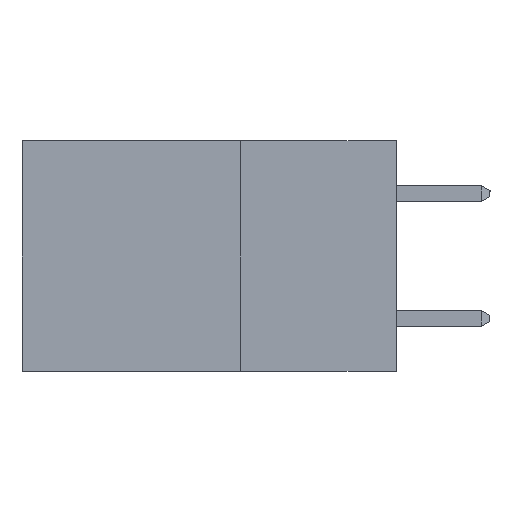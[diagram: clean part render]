
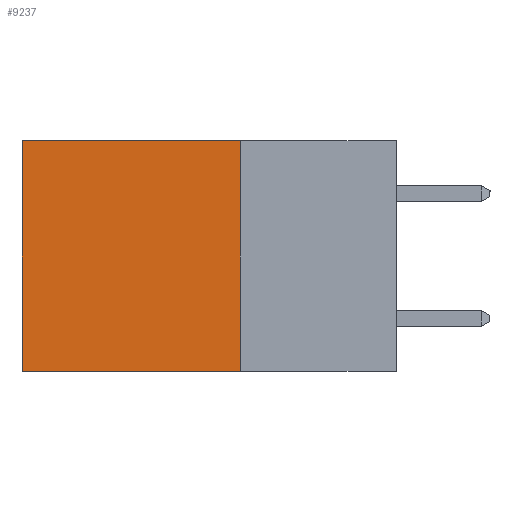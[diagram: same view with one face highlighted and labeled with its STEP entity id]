
A CAD part, left-side view. The second image highlights one B-rep face of the part: STEP entity #9237.
In plain terms, the highlighted planar face has unit normal (-1, 0, 0).
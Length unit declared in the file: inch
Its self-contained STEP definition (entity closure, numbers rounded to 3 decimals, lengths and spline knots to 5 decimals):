
#316 = DIRECTION ( 'NONE',  ( 0., 1., 0. ) ) ;
#405 = CARTESIAN_POINT ( 'NONE',  ( 0.2615, 0.25, 0. ) ) ;
#786 = AXIS2_PLACEMENT_3D ( 'NONE', #932, #842, #2247 ) ;
#842 = DIRECTION ( 'NONE',  ( 1., 0., 0. ) ) ;
#932 = CARTESIAN_POINT ( 'NONE',  ( 0.2615, 0.25, -0.37 ) ) ;
#951 = ORIENTED_EDGE ( 'NONE', *, *, #1765, .T. ) ;
#1187 = VECTOR ( 'NONE', #1898, 39.37008 ) ;
#1765 = EDGE_CURVE ( 'NONE', #8163, #3917, #7769, .T. ) ;
#1898 = DIRECTION ( 'NONE',  ( 0., 1., 0. ) ) ;
#2247 = DIRECTION ( 'NONE',  ( 0., 0., -1. ) ) ;
#2264 = EDGE_CURVE ( 'NONE', #3917, #9167, #2572, .T. ) ;
#2406 = ORIENTED_EDGE ( 'NONE', *, *, #7772, .F. ) ;
#2418 = VERTEX_POINT ( 'NONE', #7257 ) ;
#2572 = LINE ( 'NONE', #4953, #6454 ) ;
#2973 = FACE_OUTER_BOUND ( 'NONE', #7862, .T. ) ;
#3017 = CARTESIAN_POINT ( 'NONE',  ( 0.2615, 0.6, -0.37 ) ) ;
#3337 = CARTESIAN_POINT ( 'NONE',  ( 0.2615, 0.25, -0.37 ) ) ;
#3652 = EDGE_CURVE ( 'NONE', #2418, #9167, #8529, .T. ) ;
#3703 = VECTOR ( 'NONE', #5774, 39.37008 ) ;
#3917 = VERTEX_POINT ( 'NONE', #3965 ) ;
#3965 = CARTESIAN_POINT ( 'NONE',  ( 0.2615, 0.6, 0. ) ) ;
#4953 = CARTESIAN_POINT ( 'NONE',  ( 0.2615, 0.6, -0.37 ) ) ;
#5526 = ORIENTED_EDGE ( 'NONE', *, *, #3652, .F. ) ;
#5774 = DIRECTION ( 'NONE',  ( 0., 0., -1. ) ) ;
#6454 = VECTOR ( 'NONE', #7837, 39.37008 ) ;
#6478 = CARTESIAN_POINT ( 'NONE',  ( 0.2615, 0.25, 0. ) ) ;
#6488 = CARTESIAN_POINT ( 'NONE',  ( 0.2615, 0.25, -0.37 ) ) ;
#6808 = VECTOR ( 'NONE', #316, 39.37008 ) ;
#7257 = CARTESIAN_POINT ( 'NONE',  ( 0.2615, 0.25, -0.37 ) ) ;
#7401 = LINE ( 'NONE', #6488, #3703 ) ;
#7769 = LINE ( 'NONE', #405, #6808 ) ;
#7772 = EDGE_CURVE ( 'NONE', #8163, #2418, #7401, .T. ) ;
#7837 = DIRECTION ( 'NONE',  ( 0., 0., -1. ) ) ;
#7862 = EDGE_LOOP ( 'NONE', ( #8587, #5526, #2406, #951 ) ) ;
#8163 = VERTEX_POINT ( 'NONE', #6478 ) ;
#8529 = LINE ( 'NONE', #3337, #1187 ) ;
#8587 = ORIENTED_EDGE ( 'NONE', *, *, #2264, .T. ) ;
#8881 = PLANE ( 'NONE',  #786 ) ;
#9167 = VERTEX_POINT ( 'NONE', #3017 ) ;
#9237 = ADVANCED_FACE ( 'NONE', ( #2973 ), #8881, .F. ) ;
